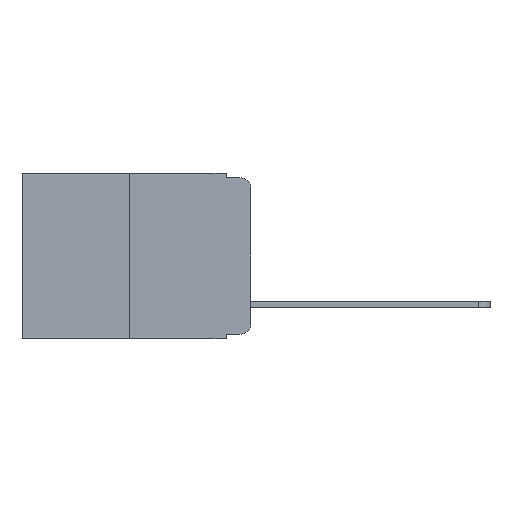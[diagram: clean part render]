
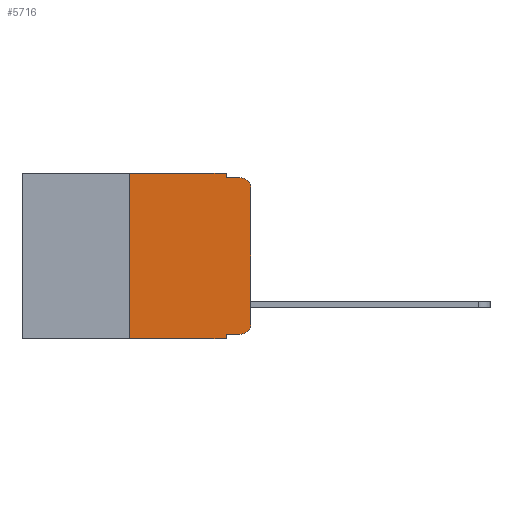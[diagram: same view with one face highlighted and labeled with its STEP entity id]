
A CAD part, left-side view. The second image highlights one B-rep face of the part: STEP entity #5716.
In plain terms, the highlighted planar face has unit normal (-1, 0, 0).
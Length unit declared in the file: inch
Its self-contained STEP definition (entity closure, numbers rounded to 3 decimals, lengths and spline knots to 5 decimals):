
#105 = DIRECTION ( 'NONE',  ( 0., 0., -1. ) ) ;
#539 = ORIENTED_EDGE ( 'NONE', *, *, #7037, .F. ) ;
#592 = DIRECTION ( 'NONE',  ( 0., -1., 0. ) ) ;
#636 = AXIS2_PLACEMENT_3D ( 'NONE', #1212, #1919, #105 ) ;
#706 = ORIENTED_EDGE ( 'NONE', *, *, #7651, .T. ) ;
#795 = LINE ( 'NONE', #13726, #11912 ) ;
#812 = LINE ( 'NONE', #13686, #11925 ) ;
#1115 = ORIENTED_EDGE ( 'NONE', *, *, #8972, .F. ) ;
#1157 = ORIENTED_EDGE ( 'NONE', *, *, #7033, .F. ) ;
#1212 = CARTESIAN_POINT ( 'NONE',  ( 0., 0.02, -0.313 ) ) ;
#1309 = ORIENTED_EDGE ( 'NONE', *, *, #6942, .F. ) ;
#1342 = ORIENTED_EDGE ( 'NONE', *, *, #6484, .T. ) ;
#1391 = CARTESIAN_POINT ( 'NONE',  ( 0., 0.473, -0.343 ) ) ;
#1618 = ORIENTED_EDGE ( 'NONE', *, *, #7056, .T. ) ;
#1665 = ORIENTED_EDGE ( 'NONE', *, *, #6394, .T. ) ;
#1694 = ORIENTED_EDGE ( 'NONE', *, *, #7055, .F. ) ;
#1919 = DIRECTION ( 'NONE',  ( -1., 0., 0. ) ) ;
#2120 = VERTEX_POINT ( 'NONE', #8606 ) ;
#2455 = CIRCLE ( 'NONE', #636, 0.02 ) ;
#2477 = CARTESIAN_POINT ( 'NONE',  ( 0., 0.051, 0. ) ) ;
#2614 = CIRCLE ( 'NONE', #7506, 0.02 ) ;
#2846 = VERTEX_POINT ( 'NONE', #11071 ) ;
#2957 = VECTOR ( 'NONE', #592, 39.37008 ) ;
#2973 = VECTOR ( 'NONE', #11256, 39.37008 ) ;
#3312 = CARTESIAN_POINT ( 'NONE',  ( 0., 0.02, -0.01 ) ) ;
#3498 = LINE ( 'NONE', #13008, #8527 ) ;
#3745 = VECTOR ( 'NONE', #8857, 39.37008 ) ;
#3881 = DIRECTION ( 'NONE',  ( 0., -1., 0. ) ) ;
#3918 = VERTEX_POINT ( 'NONE', #4523 ) ;
#3980 = FACE_OUTER_BOUND ( 'NONE', #8330, .T. ) ;
#4051 = CARTESIAN_POINT ( 'NONE',  ( 0., 0.25, -0.343 ) ) ;
#4523 = CARTESIAN_POINT ( 'NONE',  ( 0., 0.02, -0.333 ) ) ;
#4846 = AXIS2_PLACEMENT_3D ( 'NONE', #7476, #7183, #7166 ) ;
#5031 = VERTEX_POINT ( 'NONE', #3312 ) ;
#5106 = CARTESIAN_POINT ( 'NONE',  ( 0., 0., -0.313 ) ) ;
#5406 = CARTESIAN_POINT ( 'NONE',  ( 0., 0.25, 0. ) ) ;
#5716 = ADVANCED_FACE ( 'NONE', ( #3980 ), #7617, .F. ) ;
#5953 = LINE ( 'NONE', #11475, #2973 ) ;
#6394 = EDGE_CURVE ( 'NONE', #3918, #7147, #2455, .T. ) ;
#6484 = EDGE_CURVE ( 'NONE', #11711, #3918, #812, .T. ) ;
#6942 = EDGE_CURVE ( 'NONE', #11711, #2846, #795, .T. ) ;
#7033 = EDGE_CURVE ( 'NONE', #13980, #12256, #5953, .T. ) ;
#7037 = EDGE_CURVE ( 'NONE', #10675, #12106, #13573, .T. ) ;
#7055 = EDGE_CURVE ( 'NONE', #12106, #5031, #8424, .T. ) ;
#7056 = EDGE_CURVE ( 'NONE', #2120, #5031, #2614, .T. ) ;
#7058 = EDGE_CURVE ( 'NONE', #7147, #2120, #13243, .T. ) ;
#7147 = VERTEX_POINT ( 'NONE', #5106 ) ;
#7166 = DIRECTION ( 'NONE',  ( 0., 0., -1. ) ) ;
#7183 = DIRECTION ( 'NONE',  ( 1., 0., 0. ) ) ;
#7476 = CARTESIAN_POINT ( 'NONE',  ( 0., 0.473, 0. ) ) ;
#7506 = AXIS2_PLACEMENT_3D ( 'NONE', #7951, #7917, #7879 ) ;
#7617 = PLANE ( 'NONE',  #4846 ) ;
#7651 = EDGE_CURVE ( 'NONE', #13980, #2846, #8720, .T. ) ;
#7879 = DIRECTION ( 'NONE',  ( 0., 0., -1. ) ) ;
#7917 = DIRECTION ( 'NONE',  ( -1., 0., 0. ) ) ;
#7951 = CARTESIAN_POINT ( 'NONE',  ( 0., 0.02, -0.03 ) ) ;
#8114 = VECTOR ( 'NONE', #8297, 39.37008 ) ;
#8189 = CARTESIAN_POINT ( 'NONE',  ( 0., 0.051, -0.01 ) ) ;
#8252 = DIRECTION ( 'NONE',  ( 0., -1., 0. ) ) ;
#8297 = DIRECTION ( 'NONE',  ( 0., 0., 1. ) ) ;
#8330 = EDGE_LOOP ( 'NONE', ( #10705, #1618, #1694, #539, #1115, #1157, #706, #1309, #1342, #1665 ) ) ;
#8410 = CARTESIAN_POINT ( 'NONE',  ( 0., 0.051, -0.01 ) ) ;
#8424 = LINE ( 'NONE', #8189, #11038 ) ;
#8527 = VECTOR ( 'NONE', #3881, 39.37008 ) ;
#8546 = CARTESIAN_POINT ( 'NONE',  ( 0., 0.051, -0.333 ) ) ;
#8584 = CARTESIAN_POINT ( 'NONE',  ( 0., 0., 0. ) ) ;
#8606 = CARTESIAN_POINT ( 'NONE',  ( 0., 0., -0.03 ) ) ;
#8720 = LINE ( 'NONE', #1391, #2957 ) ;
#8857 = DIRECTION ( 'NONE',  ( 0., 0., -1. ) ) ;
#8972 = EDGE_CURVE ( 'NONE', #12256, #10675, #3498, .T. ) ;
#10527 = CARTESIAN_POINT ( 'NONE',  ( 0., 0.051, 0. ) ) ;
#10675 = VERTEX_POINT ( 'NONE', #2477 ) ;
#10705 = ORIENTED_EDGE ( 'NONE', *, *, #7058, .T. ) ;
#11038 = VECTOR ( 'NONE', #8252, 39.37008 ) ;
#11071 = CARTESIAN_POINT ( 'NONE',  ( 0., 0.051, -0.343 ) ) ;
#11256 = DIRECTION ( 'NONE',  ( 0., 0., 1. ) ) ;
#11475 = CARTESIAN_POINT ( 'NONE',  ( 0., 0.25, 0. ) ) ;
#11711 = VERTEX_POINT ( 'NONE', #8546 ) ;
#11912 = VECTOR ( 'NONE', #13483, 39.37008 ) ;
#11925 = VECTOR ( 'NONE', #12951, 39.37008 ) ;
#12106 = VERTEX_POINT ( 'NONE', #8410 ) ;
#12256 = VERTEX_POINT ( 'NONE', #5406 ) ;
#12951 = DIRECTION ( 'NONE',  ( 0., -1., 0. ) ) ;
#13008 = CARTESIAN_POINT ( 'NONE',  ( 0., 0.473, 0. ) ) ;
#13243 = LINE ( 'NONE', #8584, #8114 ) ;
#13483 = DIRECTION ( 'NONE',  ( 0., 0., -1. ) ) ;
#13573 = LINE ( 'NONE', #10527, #3745 ) ;
#13686 = CARTESIAN_POINT ( 'NONE',  ( 0., 0.051, -0.333 ) ) ;
#13726 = CARTESIAN_POINT ( 'NONE',  ( 0., 0.051, 0. ) ) ;
#13980 = VERTEX_POINT ( 'NONE', #4051 ) ;
